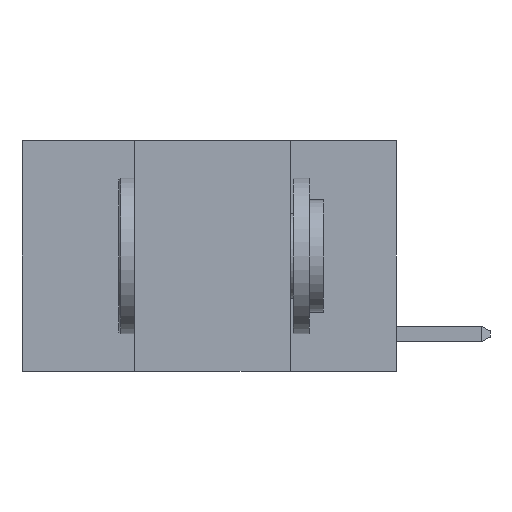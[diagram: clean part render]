
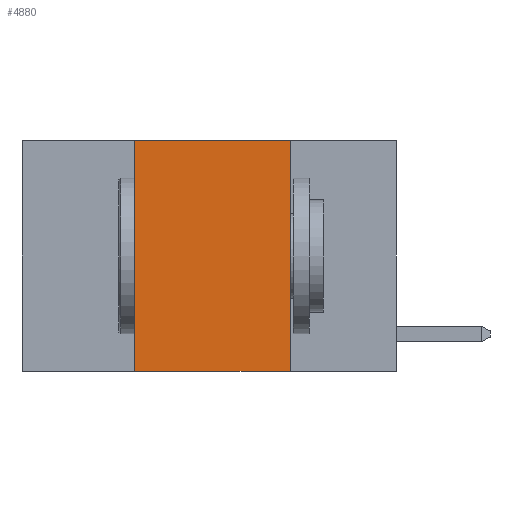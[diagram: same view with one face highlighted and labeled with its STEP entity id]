
A CAD part, left-side view. The second image highlights one B-rep face of the part: STEP entity #4880.
In plain terms, the highlighted planar face has unit normal (-1, 0, 0).
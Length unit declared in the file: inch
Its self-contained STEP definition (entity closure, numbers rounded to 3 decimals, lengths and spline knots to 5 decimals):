
#67 = LINE ( 'NONE', #3046, #9311 ) ;
#343 = EDGE_CURVE ( 'NONE', #3472, #10670, #67, .T. ) ;
#581 = ORIENTED_EDGE ( 'NONE', *, *, #10905, .F. ) ;
#1465 = DIRECTION ( 'NONE',  ( 0., 0., -1. ) ) ;
#1524 = LINE ( 'NONE', #2982, #10010 ) ;
#1590 = VECTOR ( 'NONE', #6176, 39.37008 ) ;
#1683 = ORIENTED_EDGE ( 'NONE', *, *, #3178, .F. ) ;
#1936 = VERTEX_POINT ( 'NONE', #8276 ) ;
#2075 = DIRECTION ( 'NONE',  ( 0., 0., 1. ) ) ;
#2964 = DIRECTION ( 'NONE',  ( 0., 0., -1. ) ) ;
#2982 = CARTESIAN_POINT ( 'NONE',  ( 0., 0.42, 0. ) ) ;
#2992 = VERTEX_POINT ( 'NONE', #10134 ) ;
#3046 = CARTESIAN_POINT ( 'NONE',  ( 0., 0.6, -0.37 ) ) ;
#3178 = EDGE_CURVE ( 'NONE', #1936, #2992, #10068, .T. ) ;
#3283 = PLANE ( 'NONE',  #7968 ) ;
#3472 = VERTEX_POINT ( 'NONE', #10057 ) ;
#4880 = ADVANCED_FACE ( 'NONE', ( #9666 ), #3283, .F. ) ;
#5668 = CARTESIAN_POINT ( 'NONE',  ( 0., 0.17, 0. ) ) ;
#6176 = DIRECTION ( 'NONE',  ( 0., -1., 0. ) ) ;
#6260 = LINE ( 'NONE', #5668, #6544 ) ;
#6544 = VECTOR ( 'NONE', #2964, 39.37008 ) ;
#6844 = CARTESIAN_POINT ( 'NONE',  ( 0., 0.6, 0. ) ) ;
#6884 = DIRECTION ( 'NONE',  ( 1., 0., 0. ) ) ;
#7757 = EDGE_LOOP ( 'NONE', ( #10470, #1683, #581, #11043 ) ) ;
#7968 = AXIS2_PLACEMENT_3D ( 'NONE', #6844, #6884, #1465 ) ;
#8276 = CARTESIAN_POINT ( 'NONE',  ( 0., 0.42, 0. ) ) ;
#8549 = EDGE_CURVE ( 'NONE', #2992, #10670, #6260, .T. ) ;
#8650 = CARTESIAN_POINT ( 'NONE',  ( 0., 0.17, -0.37 ) ) ;
#9311 = VECTOR ( 'NONE', #11073, 39.37008 ) ;
#9666 = FACE_OUTER_BOUND ( 'NONE', #7757, .T. ) ;
#10010 = VECTOR ( 'NONE', #2075, 39.37008 ) ;
#10057 = CARTESIAN_POINT ( 'NONE',  ( 0., 0.42, -0.37 ) ) ;
#10068 = LINE ( 'NONE', #11139, #1590 ) ;
#10134 = CARTESIAN_POINT ( 'NONE',  ( 0., 0.17, 0. ) ) ;
#10470 = ORIENTED_EDGE ( 'NONE', *, *, #8549, .F. ) ;
#10670 = VERTEX_POINT ( 'NONE', #8650 ) ;
#10905 = EDGE_CURVE ( 'NONE', #3472, #1936, #1524, .T. ) ;
#11043 = ORIENTED_EDGE ( 'NONE', *, *, #343, .T. ) ;
#11073 = DIRECTION ( 'NONE',  ( 0., -1., 0. ) ) ;
#11139 = CARTESIAN_POINT ( 'NONE',  ( 0., 0.6, 0. ) ) ;
